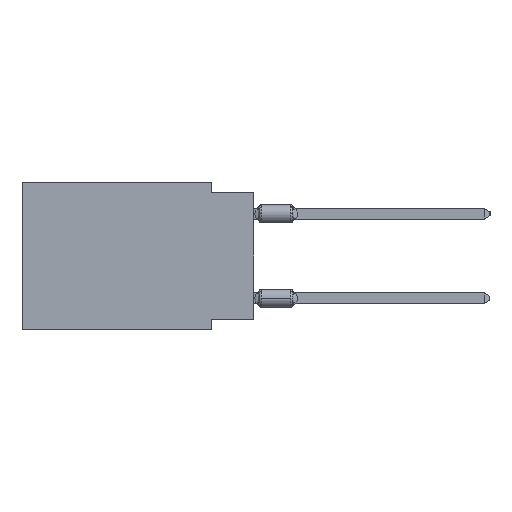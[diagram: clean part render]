
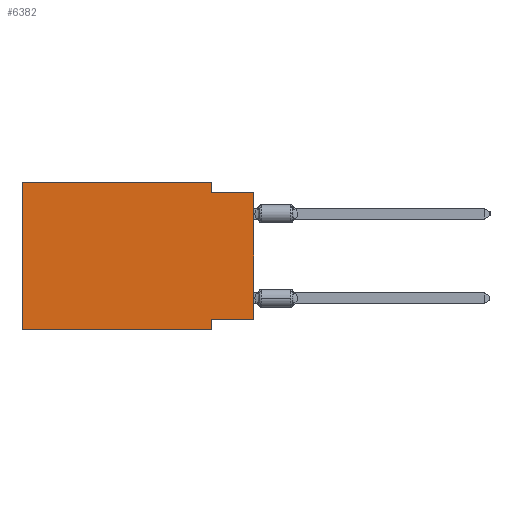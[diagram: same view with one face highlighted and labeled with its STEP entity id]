
A CAD part, left-side view. The second image highlights one B-rep face of the part: STEP entity #6382.
In plain terms, the highlighted planar face has unit normal (-1, 0, 0).
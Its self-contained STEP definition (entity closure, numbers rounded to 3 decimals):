
#3452 = DIRECTION ( 'NONE',  ( 0., 0., -1. ) ) ;
#3460 = CARTESIAN_POINT ( 'NONE',  ( 0., 2.54, -8.255 ) ) ;
#3485 = DIRECTION ( 'NONE',  ( 0., -1., 0. ) ) ;
#4440 = EDGE_CURVE ( 'NONE', #47209, #12175, #25603, .T. ) ;
#6382 = ADVANCED_FACE ( 'NONE', ( #32404 ), #49283, .F. ) ;
#7260 = DIRECTION ( 'NONE',  ( 1., 0., 0. ) ) ;
#7874 = EDGE_CURVE ( 'NONE', #29805, #12175, #27736, .T. ) ;
#8630 = ORIENTED_EDGE ( 'NONE', *, *, #47088, .F. ) ;
#9546 = VERTEX_POINT ( 'NONE', #3460 ) ;
#9796 = VECTOR ( 'NONE', #3485, 1000. ) ;
#11568 = CARTESIAN_POINT ( 'NONE',  ( 0., 13.97, 0. ) ) ;
#12175 = VERTEX_POINT ( 'NONE', #30275 ) ;
#12831 = LINE ( 'NONE', #33008, #28525 ) ;
#14293 = VECTOR ( 'NONE', #39953, 1000. ) ;
#14792 = LINE ( 'NONE', #44631, #14293 ) ;
#15834 = DIRECTION ( 'NONE',  ( 0., 0., -1. ) ) ;
#15843 = DIRECTION ( 'NONE',  ( 0., -1., 0. ) ) ;
#17256 = VERTEX_POINT ( 'NONE', #43246 ) ;
#17287 = EDGE_CURVE ( 'NONE', #26075, #46110, #44350, .T. ) ;
#17865 = ORIENTED_EDGE ( 'NONE', *, *, #40296, .F. ) ;
#18019 = VECTOR ( 'NONE', #27501, 1000. ) ;
#19022 = CARTESIAN_POINT ( 'NONE',  ( 0., 0., -8.255 ) ) ;
#19906 = LINE ( 'NONE', #49215, #33865 ) ;
#21514 = CARTESIAN_POINT ( 'NONE',  ( 0., 2.54, -8.89 ) ) ;
#23844 = EDGE_CURVE ( 'NONE', #17256, #43948, #45494, .T. ) ;
#25603 = LINE ( 'NONE', #38053, #48822 ) ;
#26075 = VERTEX_POINT ( 'NONE', #11568 ) ;
#26471 = VECTOR ( 'NONE', #32264, 1000. ) ;
#27218 = CARTESIAN_POINT ( 'NONE',  ( 0., 13.97, 0. ) ) ;
#27501 = DIRECTION ( 'NONE',  ( 0., -1., 0. ) ) ;
#27736 = LINE ( 'NONE', #36300, #48978 ) ;
#28525 = VECTOR ( 'NONE', #3452, 1000. ) ;
#29805 = VERTEX_POINT ( 'NONE', #31141 ) ;
#30275 = CARTESIAN_POINT ( 'NONE',  ( 0., 0., -0.635 ) ) ;
#31141 = CARTESIAN_POINT ( 'NONE',  ( 0., 2.54, -0.635 ) ) ;
#32264 = DIRECTION ( 'NONE',  ( 0., 1., 0. ) ) ;
#32404 = FACE_OUTER_BOUND ( 'NONE', #53157, .T. ) ;
#33008 = CARTESIAN_POINT ( 'NONE',  ( 0., 2.54, -8.89 ) ) ;
#33349 = DIRECTION ( 'NONE',  ( 0., 0., 1. ) ) ;
#33422 = ORIENTED_EDGE ( 'NONE', *, *, #4440, .T. ) ;
#33865 = VECTOR ( 'NONE', #53098, 1000. ) ;
#34551 = ORIENTED_EDGE ( 'NONE', *, *, #23844, .T. ) ;
#36300 = CARTESIAN_POINT ( 'NONE',  ( 0., 0., -0.635 ) ) ;
#38053 = CARTESIAN_POINT ( 'NONE',  ( 0., 0., 0. ) ) ;
#39953 = DIRECTION ( 'NONE',  ( 0., 0., 1. ) ) ;
#40296 = EDGE_CURVE ( 'NONE', #47209, #9546, #44428, .T. ) ;
#40684 = ORIENTED_EDGE ( 'NONE', *, *, #17287, .F. ) ;
#41081 = CARTESIAN_POINT ( 'NONE',  ( 0., 13.97, -8.89 ) ) ;
#42661 = CARTESIAN_POINT ( 'NONE',  ( 0., 0., -8.255 ) ) ;
#43246 = CARTESIAN_POINT ( 'NONE',  ( 0., 13.97, -8.89 ) ) ;
#43948 = VERTEX_POINT ( 'NONE', #21514 ) ;
#44350 = LINE ( 'NONE', #27218, #18019 ) ;
#44428 = LINE ( 'NONE', #19022, #26471 ) ;
#44631 = CARTESIAN_POINT ( 'NONE',  ( 0., 13.97, 0. ) ) ;
#44975 = ORIENTED_EDGE ( 'NONE', *, *, #7874, .F. ) ;
#45127 = CARTESIAN_POINT ( 'NONE',  ( 0., 13.97, 0. ) ) ;
#45494 = LINE ( 'NONE', #41081, #9796 ) ;
#45512 = ORIENTED_EDGE ( 'NONE', *, *, #51457, .F. ) ;
#45733 = EDGE_CURVE ( 'NONE', #17256, #26075, #14792, .T. ) ;
#46110 = VERTEX_POINT ( 'NONE', #50723 ) ;
#47088 = EDGE_CURVE ( 'NONE', #9546, #43948, #12831, .T. ) ;
#47209 = VERTEX_POINT ( 'NONE', #42661 ) ;
#48822 = VECTOR ( 'NONE', #33349, 1000. ) ;
#48978 = VECTOR ( 'NONE', #15843, 1000. ) ;
#49215 = CARTESIAN_POINT ( 'NONE',  ( 0., 2.54, 0. ) ) ;
#49283 = PLANE ( 'NONE',  #49884 ) ;
#49884 = AXIS2_PLACEMENT_3D ( 'NONE', #45127, #7260, #15834 ) ;
#50723 = CARTESIAN_POINT ( 'NONE',  ( 0., 2.54, 0. ) ) ;
#51457 = EDGE_CURVE ( 'NONE', #46110, #29805, #19906, .T. ) ;
#52279 = ORIENTED_EDGE ( 'NONE', *, *, #45733, .F. ) ;
#53098 = DIRECTION ( 'NONE',  ( 0., 0., -1. ) ) ;
#53157 = EDGE_LOOP ( 'NONE', ( #33422, #44975, #45512, #40684, #52279, #34551, #8630, #17865 ) ) ;
